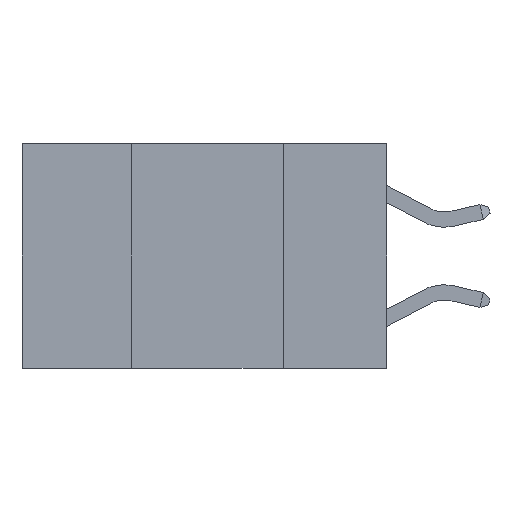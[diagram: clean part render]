
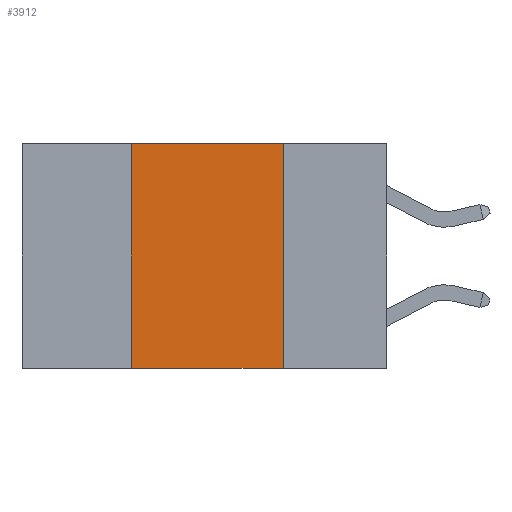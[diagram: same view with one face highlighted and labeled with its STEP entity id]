
A CAD part, left-side view. The second image highlights one B-rep face of the part: STEP entity #3912.
In plain terms, the highlighted planar face has unit normal (-1, 0, 0).
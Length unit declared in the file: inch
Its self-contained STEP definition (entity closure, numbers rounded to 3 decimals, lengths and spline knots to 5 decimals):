
#206 = VERTEX_POINT ( 'NONE', #2846 ) ;
#552 = CARTESIAN_POINT ( 'NONE',  ( 0., 0.17, 0. ) ) ;
#725 = DIRECTION ( 'NONE',  ( 0., 0., 1. ) ) ;
#797 = LINE ( 'NONE', #5518, #9626 ) ;
#895 = EDGE_CURVE ( 'NONE', #1086, #206, #797, .T. ) ;
#917 = CARTESIAN_POINT ( 'NONE',  ( 0., 0.17, 0. ) ) ;
#1086 = VERTEX_POINT ( 'NONE', #5055 ) ;
#1951 = LINE ( 'NONE', #917, #10334 ) ;
#2228 = DIRECTION ( 'NONE',  ( 0., 0., -1. ) ) ;
#2431 = LINE ( 'NONE', #6958, #11947 ) ;
#2846 = CARTESIAN_POINT ( 'NONE',  ( 0., 0.42, 0. ) ) ;
#3912 = ADVANCED_FACE ( 'NONE', ( #4354 ), #7615, .F. ) ;
#4354 = FACE_OUTER_BOUND ( 'NONE', #5082, .T. ) ;
#4954 = ORIENTED_EDGE ( 'NONE', *, *, #895, .F. ) ;
#5002 = DIRECTION ( 'NONE',  ( 0., -1., 0. ) ) ;
#5055 = CARTESIAN_POINT ( 'NONE',  ( 0., 0.42, -0.37 ) ) ;
#5082 = EDGE_LOOP ( 'NONE', ( #7848, #10036, #4954, #10589 ) ) ;
#5393 = DIRECTION ( 'NONE',  ( 0., 0., -1. ) ) ;
#5518 = CARTESIAN_POINT ( 'NONE',  ( 0., 0.42, 0. ) ) ;
#5864 = DIRECTION ( 'NONE',  ( 0., -1., 0. ) ) ;
#6954 = AXIS2_PLACEMENT_3D ( 'NONE', #8888, #12064, #5393 ) ;
#6958 = CARTESIAN_POINT ( 'NONE',  ( 0., 0.6, 0. ) ) ;
#7615 = PLANE ( 'NONE',  #6954 ) ;
#7848 = ORIENTED_EDGE ( 'NONE', *, *, #9998, .F. ) ;
#8453 = VECTOR ( 'NONE', #5002, 39.37008 ) ;
#8491 = EDGE_CURVE ( 'NONE', #1086, #8513, #9376, .T. ) ;
#8513 = VERTEX_POINT ( 'NONE', #12784 ) ;
#8888 = CARTESIAN_POINT ( 'NONE',  ( 0., 0.6, 0. ) ) ;
#9376 = LINE ( 'NONE', #12853, #8453 ) ;
#9456 = EDGE_CURVE ( 'NONE', #206, #11146, #2431, .T. ) ;
#9626 = VECTOR ( 'NONE', #725, 39.37008 ) ;
#9998 = EDGE_CURVE ( 'NONE', #11146, #8513, #1951, .T. ) ;
#10036 = ORIENTED_EDGE ( 'NONE', *, *, #9456, .F. ) ;
#10334 = VECTOR ( 'NONE', #2228, 39.37008 ) ;
#10589 = ORIENTED_EDGE ( 'NONE', *, *, #8491, .T. ) ;
#11146 = VERTEX_POINT ( 'NONE', #552 ) ;
#11947 = VECTOR ( 'NONE', #5864, 39.37008 ) ;
#12064 = DIRECTION ( 'NONE',  ( 1., 0., 0. ) ) ;
#12784 = CARTESIAN_POINT ( 'NONE',  ( 0., 0.17, -0.37 ) ) ;
#12853 = CARTESIAN_POINT ( 'NONE',  ( 0., 0.6, -0.37 ) ) ;
